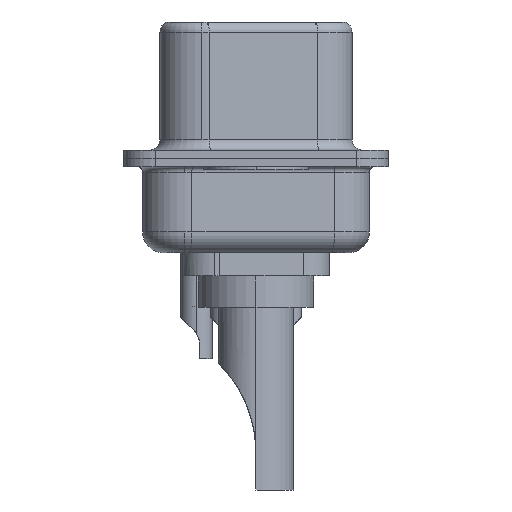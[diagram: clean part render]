
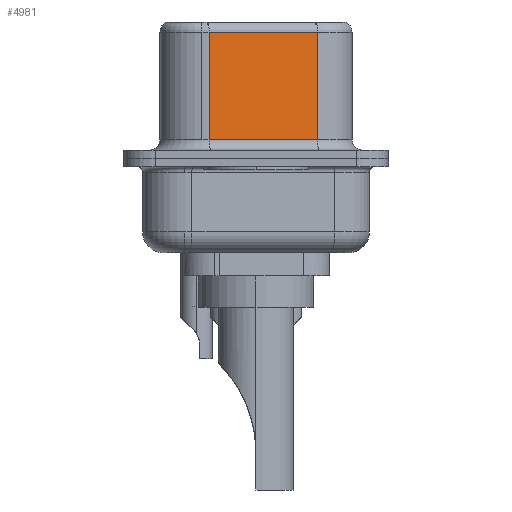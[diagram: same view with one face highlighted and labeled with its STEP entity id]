
A CAD part, left-side view. The second image highlights one B-rep face of the part: STEP entity #4981.
In plain terms, the highlighted planar face has unit normal (-0.985, -0.174, 0).
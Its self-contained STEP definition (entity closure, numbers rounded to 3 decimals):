
#686 = CARTESIAN_POINT ( 'NONE',  ( 4.58, -2.927, 6.02 ) ) ;
#1233 = AXIS2_PLACEMENT_3D ( 'NONE', #12634, #2280, #18199 ) ;
#1635 = EDGE_LOOP ( 'NONE', ( #9629, #14389, #16625, #15434 ) ) ;
#2207 = CARTESIAN_POINT ( 'NONE',  ( 3.67, 2.233, 0.9 ) ) ;
#2280 = DIRECTION ( 'NONE',  ( 0.985, 0.174, 0. ) ) ;
#2455 = PLANE ( 'NONE',  #1233 ) ;
#2681 = DIRECTION ( 'NONE',  ( 0., 0., -1. ) ) ;
#2837 = DIRECTION ( 'NONE',  ( 0., 0., -1. ) ) ;
#3058 = LINE ( 'NONE', #17310, #14051 ) ;
#4347 = LINE ( 'NONE', #12719, #7701 ) ;
#4884 = VERTEX_POINT ( 'NONE', #2207 ) ;
#4981 = ADVANCED_FACE ( 'NONE', ( #12349 ), #2455, .F. ) ;
#5670 = CARTESIAN_POINT ( 'NONE',  ( 4.58, -2.927, 6.52 ) ) ;
#6002 = EDGE_CURVE ( 'NONE', #4884, #16595, #8495, .T. ) ;
#7625 = LINE ( 'NONE', #5670, #18804 ) ;
#7701 = VECTOR ( 'NONE', #2681, 1000. ) ;
#7963 = VERTEX_POINT ( 'NONE', #686 ) ;
#8495 = LINE ( 'NONE', #8549, #16290 ) ;
#8549 = CARTESIAN_POINT ( 'NONE',  ( 4.58, -2.927, 0.9 ) ) ;
#9629 = ORIENTED_EDGE ( 'NONE', *, *, #14578, .F. ) ;
#10478 = EDGE_CURVE ( 'NONE', #13887, #4884, #4347, .T. ) ;
#11194 = EDGE_CURVE ( 'NONE', #7963, #13887, #3058, .T. ) ;
#11418 = DIRECTION ( 'NONE',  ( -0.174, 0.985, 0. ) ) ;
#12349 = FACE_OUTER_BOUND ( 'NONE', #1635, .T. ) ;
#12634 = CARTESIAN_POINT ( 'NONE',  ( 4.58, -2.927, 6.52 ) ) ;
#12719 = CARTESIAN_POINT ( 'NONE',  ( 3.67, 2.233, 6.52 ) ) ;
#13510 = DIRECTION ( 'NONE',  ( 0.174, -0.985, 0. ) ) ;
#13887 = VERTEX_POINT ( 'NONE', #18776 ) ;
#14051 = VECTOR ( 'NONE', #11418, 1000. ) ;
#14389 = ORIENTED_EDGE ( 'NONE', *, *, #11194, .T. ) ;
#14578 = EDGE_CURVE ( 'NONE', #7963, #16595, #7625, .T. ) ;
#14638 = CARTESIAN_POINT ( 'NONE',  ( 4.58, -2.927, 0.9 ) ) ;
#15434 = ORIENTED_EDGE ( 'NONE', *, *, #6002, .T. ) ;
#16290 = VECTOR ( 'NONE', #13510, 1000. ) ;
#16595 = VERTEX_POINT ( 'NONE', #14638 ) ;
#16625 = ORIENTED_EDGE ( 'NONE', *, *, #10478, .T. ) ;
#17310 = CARTESIAN_POINT ( 'NONE',  ( 4.58, -2.927, 6.02 ) ) ;
#18199 = DIRECTION ( 'NONE',  ( -0.174, 0.985, 0. ) ) ;
#18776 = CARTESIAN_POINT ( 'NONE',  ( 3.67, 2.233, 6.02 ) ) ;
#18804 = VECTOR ( 'NONE', #2837, 1000. ) ;
